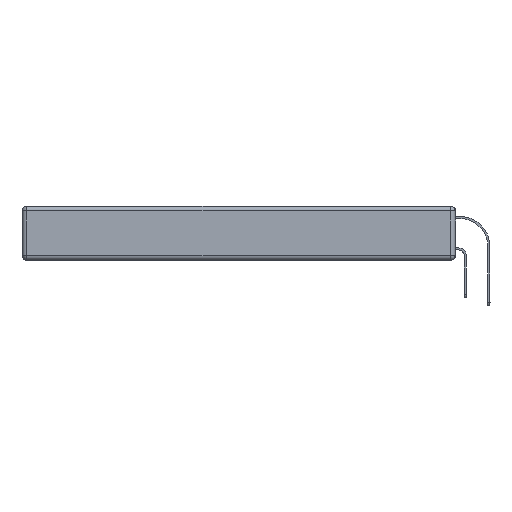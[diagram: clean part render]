
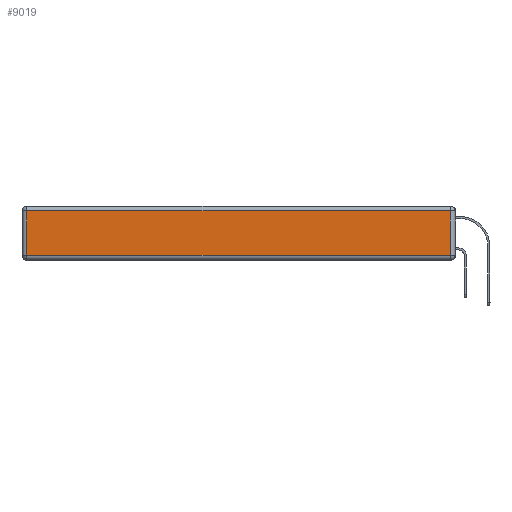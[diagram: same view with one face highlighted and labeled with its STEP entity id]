
A CAD part, left-side view. The second image highlights one B-rep face of the part: STEP entity #9019.
In plain terms, the highlighted planar face has unit normal (-1, 0, 0).
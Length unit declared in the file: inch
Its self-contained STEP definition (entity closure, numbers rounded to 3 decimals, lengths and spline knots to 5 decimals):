
#1277 = LINE ( 'NONE', #5773, #20011 ) ;
#3425 = DIRECTION ( 'NONE',  ( 0., -1., 0. ) ) ;
#4712 = EDGE_CURVE ( 'NONE', #8242, #26595, #27667, .T. ) ;
#5139 = VECTOR ( 'NONE', #25928, 39.37008 ) ;
#5773 = CARTESIAN_POINT ( 'NONE',  ( 0., 0.03, -0.343 ) ) ;
#6118 = EDGE_CURVE ( 'NONE', #26595, #15077, #23512, .T. ) ;
#6293 = CARTESIAN_POINT ( 'NONE',  ( 0., 0.03, -0.313 ) ) ;
#7188 = AXIS2_PLACEMENT_3D ( 'NONE', #20238, #27022, #22688 ) ;
#7236 = PLANE ( 'NONE',  #7188 ) ;
#7433 = CARTESIAN_POINT ( 'NONE',  ( 0., 2.72, -0.343 ) ) ;
#7784 = CARTESIAN_POINT ( 'NONE',  ( 0., 2.72, -0.313 ) ) ;
#8166 = VECTOR ( 'NONE', #3425, 39.37008 ) ;
#8242 = VERTEX_POINT ( 'NONE', #9311 ) ;
#8307 = CARTESIAN_POINT ( 'NONE',  ( 0., 2.75, -0.03 ) ) ;
#9019 = ADVANCED_FACE ( 'NONE', ( #18083 ), #7236, .T. ) ;
#9311 = CARTESIAN_POINT ( 'NONE',  ( 0., 2.72, -0.03 ) ) ;
#10237 = ORIENTED_EDGE ( 'NONE', *, *, #10245, .T. ) ;
#10245 = EDGE_CURVE ( 'NONE', #17722, #8242, #10601, .T. ) ;
#10601 = LINE ( 'NONE', #8307, #5139 ) ;
#12545 = DIRECTION ( 'NONE',  ( 0., 0., 1. ) ) ;
#13277 = CARTESIAN_POINT ( 'NONE',  ( 0., 0.03, -0.03 ) ) ;
#15077 = VERTEX_POINT ( 'NONE', #6293 ) ;
#16882 = CARTESIAN_POINT ( 'NONE',  ( 0., 0., -0.313 ) ) ;
#17722 = VERTEX_POINT ( 'NONE', #13277 ) ;
#18083 = FACE_OUTER_BOUND ( 'NONE', #18852, .T. ) ;
#18852 = EDGE_LOOP ( 'NONE', ( #27216, #27198, #10237, #19464 ) ) ;
#19464 = ORIENTED_EDGE ( 'NONE', *, *, #4712, .T. ) ;
#20011 = VECTOR ( 'NONE', #12545, 39.37008 ) ;
#20238 = CARTESIAN_POINT ( 'NONE',  ( 0., 0., -0.343 ) ) ;
#20441 = EDGE_CURVE ( 'NONE', #15077, #17722, #1277, .T. ) ;
#22688 = DIRECTION ( 'NONE',  ( 0., 0., 1. ) ) ;
#23512 = LINE ( 'NONE', #16882, #8166 ) ;
#24343 = VECTOR ( 'NONE', #25214, 39.37008 ) ;
#25214 = DIRECTION ( 'NONE',  ( 0., 0., -1. ) ) ;
#25928 = DIRECTION ( 'NONE',  ( 0., 1., 0. ) ) ;
#26595 = VERTEX_POINT ( 'NONE', #7784 ) ;
#27022 = DIRECTION ( 'NONE',  ( -1., 0., 0. ) ) ;
#27198 = ORIENTED_EDGE ( 'NONE', *, *, #20441, .T. ) ;
#27216 = ORIENTED_EDGE ( 'NONE', *, *, #6118, .T. ) ;
#27667 = LINE ( 'NONE', #7433, #24343 ) ;
